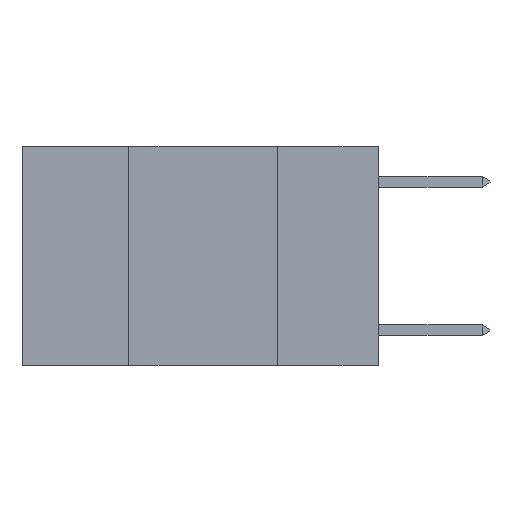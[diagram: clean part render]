
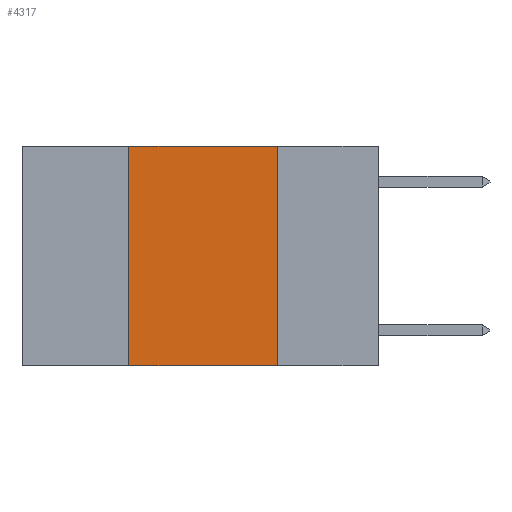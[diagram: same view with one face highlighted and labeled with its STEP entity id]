
A CAD part, left-side view. The second image highlights one B-rep face of the part: STEP entity #4317.
In plain terms, the highlighted planar face has unit normal (-1, 0, 0).
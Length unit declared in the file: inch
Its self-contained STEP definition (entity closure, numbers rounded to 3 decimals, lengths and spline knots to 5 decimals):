
#640 = VERTEX_POINT ( 'NONE', #2786 ) ;
#968 = VECTOR ( 'NONE', #5530, 39.37008 ) ;
#1515 = CARTESIAN_POINT ( 'NONE',  ( 0., 0.17, 0. ) ) ;
#1522 = LINE ( 'NONE', #3123, #6987 ) ;
#1678 = ORIENTED_EDGE ( 'NONE', *, *, #6889, .F. ) ;
#2317 = FACE_OUTER_BOUND ( 'NONE', #6218, .T. ) ;
#2409 = DIRECTION ( 'NONE',  ( 0., 0., 1. ) ) ;
#2474 = VERTEX_POINT ( 'NONE', #5634 ) ;
#2786 = CARTESIAN_POINT ( 'NONE',  ( 0., 0.42, 0. ) ) ;
#2998 = LINE ( 'NONE', #6867, #968 ) ;
#3123 = CARTESIAN_POINT ( 'NONE',  ( 0., 0.42, 0. ) ) ;
#3149 = CARTESIAN_POINT ( 'NONE',  ( 0., 0.6, 0. ) ) ;
#3471 = VECTOR ( 'NONE', #3982, 39.37008 ) ;
#3583 = ORIENTED_EDGE ( 'NONE', *, *, #7736, .T. ) ;
#3599 = DIRECTION ( 'NONE',  ( 0., 0., -1. ) ) ;
#3982 = DIRECTION ( 'NONE',  ( 0., -1., 0. ) ) ;
#4142 = VERTEX_POINT ( 'NONE', #5346 ) ;
#4317 = ADVANCED_FACE ( 'NONE', ( #2317 ), #7116, .F. ) ;
#5163 = EDGE_CURVE ( 'NONE', #640, #2474, #5893, .T. ) ;
#5318 = VERTEX_POINT ( 'NONE', #6895 ) ;
#5346 = CARTESIAN_POINT ( 'NONE',  ( 0., 0.17, -0.37 ) ) ;
#5478 = VECTOR ( 'NONE', #6581, 39.37008 ) ;
#5530 = DIRECTION ( 'NONE',  ( 0., -1., 0. ) ) ;
#5634 = CARTESIAN_POINT ( 'NONE',  ( 0., 0.17, 0. ) ) ;
#5794 = CARTESIAN_POINT ( 'NONE',  ( 0., 0.6, 0. ) ) ;
#5893 = LINE ( 'NONE', #3149, #3471 ) ;
#5917 = ORIENTED_EDGE ( 'NONE', *, *, #5163, .F. ) ;
#6218 = EDGE_LOOP ( 'NONE', ( #7565, #5917, #1678, #3583 ) ) ;
#6553 = AXIS2_PLACEMENT_3D ( 'NONE', #5794, #7759, #3599 ) ;
#6581 = DIRECTION ( 'NONE',  ( 0., 0., -1. ) ) ;
#6867 = CARTESIAN_POINT ( 'NONE',  ( 0., 0.6, -0.37 ) ) ;
#6889 = EDGE_CURVE ( 'NONE', #5318, #640, #1522, .T. ) ;
#6895 = CARTESIAN_POINT ( 'NONE',  ( 0., 0.42, -0.37 ) ) ;
#6987 = VECTOR ( 'NONE', #2409, 39.37008 ) ;
#7116 = PLANE ( 'NONE',  #6553 ) ;
#7266 = LINE ( 'NONE', #1515, #5478 ) ;
#7565 = ORIENTED_EDGE ( 'NONE', *, *, #8194, .F. ) ;
#7736 = EDGE_CURVE ( 'NONE', #5318, #4142, #2998, .T. ) ;
#7759 = DIRECTION ( 'NONE',  ( 1., 0., 0. ) ) ;
#8194 = EDGE_CURVE ( 'NONE', #2474, #4142, #7266, .T. ) ;
